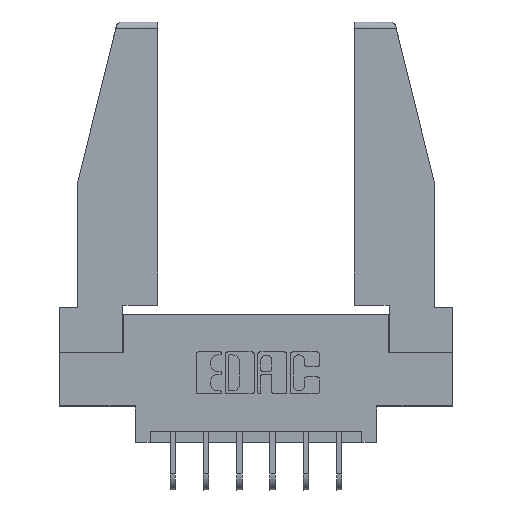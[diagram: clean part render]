
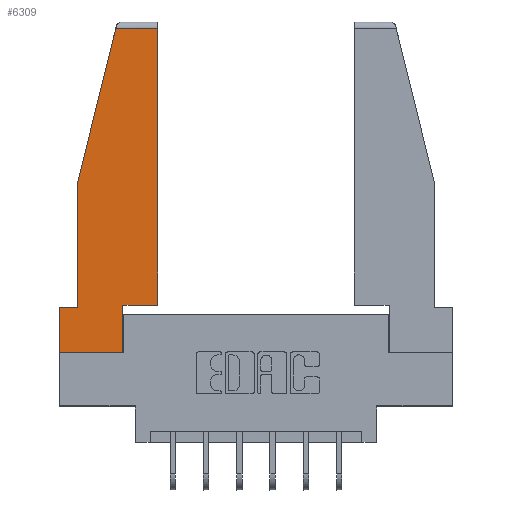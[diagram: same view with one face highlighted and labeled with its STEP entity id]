
A CAD part, top view. The second image highlights one B-rep face of the part: STEP entity #6309.
In plain terms, the highlighted planar face has unit normal (0, 0, 1).
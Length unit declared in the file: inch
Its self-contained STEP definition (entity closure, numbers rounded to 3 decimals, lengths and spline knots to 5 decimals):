
#50 = VECTOR ( 'NONE', #6775, 39.37008 ) ;
#431 = LINE ( 'NONE', #9553, #3019 ) ;
#507 = CARTESIAN_POINT ( 'NONE',  ( 0.297, 0., 0. ) ) ;
#559 = VECTOR ( 'NONE', #1677, 39.37008 ) ;
#875 = VECTOR ( 'NONE', #3894, 39.37008 ) ;
#1325 = EDGE_CURVE ( 'NONE', #7231, #12982, #431, .T. ) ;
#1499 = EDGE_CURVE ( 'NONE', #11560, #1856, #12467, .T. ) ;
#1677 = DIRECTION ( 'NONE',  ( -0.239, -0.971, 0. ) ) ;
#1856 = VERTEX_POINT ( 'NONE', #11350 ) ;
#1923 = VERTEX_POINT ( 'NONE', #1951 ) ;
#1951 = CARTESIAN_POINT ( 'NONE',  ( 0.461, 0.223, 0. ) ) ;
#2062 = ORIENTED_EDGE ( 'NONE', *, *, #10388, .T. ) ;
#2611 = CARTESIAN_POINT ( 'NONE',  ( 0., 1.52, 0. ) ) ;
#2771 = DIRECTION ( 'NONE',  ( 1., 0., 0. ) ) ;
#2800 = CARTESIAN_POINT ( 'NONE',  ( 0.461, 1.52, 0. ) ) ;
#2828 = LINE ( 'NONE', #12039, #50 ) ;
#2857 = VECTOR ( 'NONE', #10008, 39.37008 ) ;
#2955 = DIRECTION ( 'NONE',  ( 0., 0., 1. ) ) ;
#3019 = VECTOR ( 'NONE', #9767, 39.37008 ) ;
#3586 = CARTESIAN_POINT ( 'NONE',  ( 0.086, 0.21, 0. ) ) ;
#3832 = EDGE_CURVE ( 'NONE', #1856, #7405, #13466, .T. ) ;
#3894 = DIRECTION ( 'NONE',  ( 1., 0., 0. ) ) ;
#4003 = CARTESIAN_POINT ( 'NONE',  ( 0.086, 0.8, 0. ) ) ;
#4020 = ORIENTED_EDGE ( 'NONE', *, *, #8757, .T. ) ;
#4048 = EDGE_LOOP ( 'NONE', ( #7773, #8684, #11435, #4020, #2062, #13103, #11301, #6444, #8760 ) ) ;
#4239 = CARTESIAN_POINT ( 'NONE',  ( 0., 0.21, 0. ) ) ;
#4478 = DIRECTION ( 'NONE',  ( -1., 0., 0. ) ) ;
#4914 = AXIS2_PLACEMENT_3D ( 'NONE', #11475, #2955, #10381 ) ;
#5029 = VERTEX_POINT ( 'NONE', #507 ) ;
#5956 = VERTEX_POINT ( 'NONE', #3586 ) ;
#6276 = PLANE ( 'NONE',  #4914 ) ;
#6309 = ADVANCED_FACE ( 'NONE', ( #12851 ), #6276, .T. ) ;
#6327 = DIRECTION ( 'NONE',  ( 0., -1., 0. ) ) ;
#6444 = ORIENTED_EDGE ( 'NONE', *, *, #7722, .T. ) ;
#6702 = LINE ( 'NONE', #7091, #7863 ) ;
#6775 = DIRECTION ( 'NONE',  ( 0., 1., 0. ) ) ;
#6817 = EDGE_CURVE ( 'NONE', #8862, #1923, #6702, .T. ) ;
#7091 = CARTESIAN_POINT ( 'NONE',  ( 0.297, 0.223, 0. ) ) ;
#7168 = VECTOR ( 'NONE', #6327, 39.37008 ) ;
#7211 = LINE ( 'NONE', #4239, #12312 ) ;
#7231 = VERTEX_POINT ( 'NONE', #12670 ) ;
#7405 = VERTEX_POINT ( 'NONE', #4003 ) ;
#7692 = DIRECTION ( 'NONE',  ( 0., 1., 0. ) ) ;
#7722 = EDGE_CURVE ( 'NONE', #5029, #8862, #9497, .T. ) ;
#7773 = ORIENTED_EDGE ( 'NONE', *, *, #12106, .T. ) ;
#7863 = VECTOR ( 'NONE', #2771, 39.37008 ) ;
#8342 = CARTESIAN_POINT ( 'NONE',  ( 0.297, 0.223, 0. ) ) ;
#8680 = CARTESIAN_POINT ( 'NONE',  ( 0.297, 0., 0. ) ) ;
#8684 = ORIENTED_EDGE ( 'NONE', *, *, #1499, .T. ) ;
#8757 = EDGE_CURVE ( 'NONE', #7405, #5956, #9947, .T. ) ;
#8760 = ORIENTED_EDGE ( 'NONE', *, *, #6817, .T. ) ;
#8862 = VERTEX_POINT ( 'NONE', #8342 ) ;
#9497 = LINE ( 'NONE', #8680, #12165 ) ;
#9553 = CARTESIAN_POINT ( 'NONE',  ( 0., 0.21, 0. ) ) ;
#9767 = DIRECTION ( 'NONE',  ( 0., -1., 0. ) ) ;
#9947 = LINE ( 'NONE', #11581, #7168 ) ;
#10008 = DIRECTION ( 'NONE',  ( -1., 0., 0. ) ) ;
#10031 = CARTESIAN_POINT ( 'NONE',  ( 0., 0., 0. ) ) ;
#10091 = LINE ( 'NONE', #10398, #875 ) ;
#10381 = DIRECTION ( 'NONE',  ( 1., 0., 0. ) ) ;
#10388 = EDGE_CURVE ( 'NONE', #5956, #7231, #7211, .T. ) ;
#10398 = CARTESIAN_POINT ( 'NONE',  ( 0., 0., 0. ) ) ;
#11070 = CARTESIAN_POINT ( 'NONE',  ( 0.271, 1.55, 0. ) ) ;
#11301 = ORIENTED_EDGE ( 'NONE', *, *, #12734, .T. ) ;
#11350 = CARTESIAN_POINT ( 'NONE',  ( 0.2636, 1.52, 0. ) ) ;
#11435 = ORIENTED_EDGE ( 'NONE', *, *, #3832, .T. ) ;
#11475 = CARTESIAN_POINT ( 'NONE',  ( 0., 0., 0. ) ) ;
#11560 = VERTEX_POINT ( 'NONE', #2800 ) ;
#11581 = CARTESIAN_POINT ( 'NONE',  ( 0.086, 0.8, 0. ) ) ;
#12039 = CARTESIAN_POINT ( 'NONE',  ( 0.461, 0.223, 0. ) ) ;
#12106 = EDGE_CURVE ( 'NONE', #1923, #11560, #2828, .T. ) ;
#12165 = VECTOR ( 'NONE', #7692, 39.37008 ) ;
#12312 = VECTOR ( 'NONE', #4478, 39.37008 ) ;
#12467 = LINE ( 'NONE', #2611, #2857 ) ;
#12670 = CARTESIAN_POINT ( 'NONE',  ( 0., 0.21, 0. ) ) ;
#12734 = EDGE_CURVE ( 'NONE', #12982, #5029, #10091, .T. ) ;
#12851 = FACE_OUTER_BOUND ( 'NONE', #4048, .T. ) ;
#12982 = VERTEX_POINT ( 'NONE', #10031 ) ;
#13103 = ORIENTED_EDGE ( 'NONE', *, *, #1325, .T. ) ;
#13466 = LINE ( 'NONE', #11070, #559 ) ;
